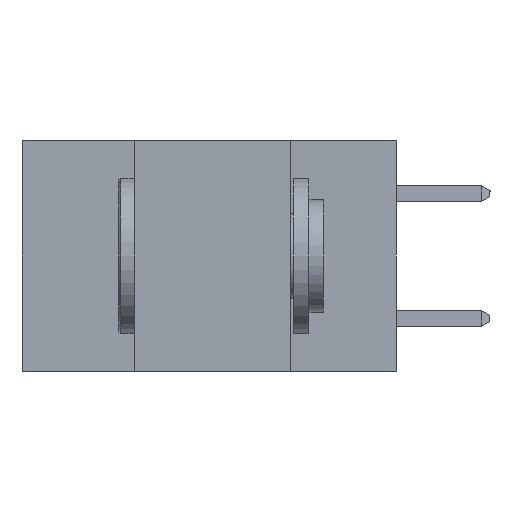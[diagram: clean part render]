
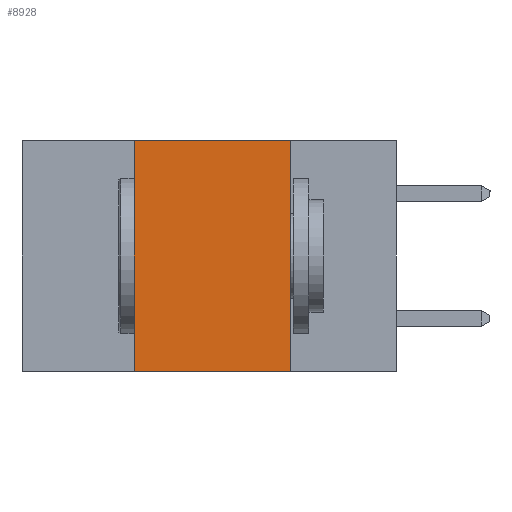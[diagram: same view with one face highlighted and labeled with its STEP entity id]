
A CAD part, left-side view. The second image highlights one B-rep face of the part: STEP entity #8928.
In plain terms, the highlighted planar face has unit normal (-1, 0, 0).
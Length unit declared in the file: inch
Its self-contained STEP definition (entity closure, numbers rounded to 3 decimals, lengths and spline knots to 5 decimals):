
#382 = EDGE_LOOP ( 'NONE', ( #12655, #15181, #7076, #5260 ) ) ;
#441 = VERTEX_POINT ( 'NONE', #9304 ) ;
#1180 = LINE ( 'NONE', #4933, #10960 ) ;
#1474 = VECTOR ( 'NONE', #10376, 39.37008 ) ;
#1528 = CARTESIAN_POINT ( 'NONE',  ( 0., 0.6, 0. ) ) ;
#1882 = AXIS2_PLACEMENT_3D ( 'NONE', #14109, #8125, #6566 ) ;
#2061 = DIRECTION ( 'NONE',  ( 0., 0., -1. ) ) ;
#2540 = LINE ( 'NONE', #1528, #10389 ) ;
#2710 = EDGE_CURVE ( 'NONE', #3416, #14634, #12738, .T. ) ;
#3416 = VERTEX_POINT ( 'NONE', #5160 ) ;
#3447 = DIRECTION ( 'NONE',  ( 0., -1., 0. ) ) ;
#4645 = CARTESIAN_POINT ( 'NONE',  ( 0., 0.42, 0. ) ) ;
#4933 = CARTESIAN_POINT ( 'NONE',  ( 0., 0.6, -0.37 ) ) ;
#5160 = CARTESIAN_POINT ( 'NONE',  ( 0., 0.42, -0.37 ) ) ;
#5260 = ORIENTED_EDGE ( 'NONE', *, *, #10572, .T. ) ;
#5879 = VECTOR ( 'NONE', #2061, 39.37008 ) ;
#6272 = EDGE_CURVE ( 'NONE', #441, #8677, #11792, .T. ) ;
#6566 = DIRECTION ( 'NONE',  ( 0., 0., -1. ) ) ;
#6716 = PLANE ( 'NONE',  #1882 ) ;
#7076 = ORIENTED_EDGE ( 'NONE', *, *, #2710, .F. ) ;
#7812 = EDGE_CURVE ( 'NONE', #14634, #441, #2540, .T. ) ;
#8125 = DIRECTION ( 'NONE',  ( 1., 0., 0. ) ) ;
#8677 = VERTEX_POINT ( 'NONE', #13109 ) ;
#8928 = ADVANCED_FACE ( 'NONE', ( #11424 ), #6716, .F. ) ;
#9304 = CARTESIAN_POINT ( 'NONE',  ( 0., 0.17, 0. ) ) ;
#10376 = DIRECTION ( 'NONE',  ( 0., 0., 1. ) ) ;
#10389 = VECTOR ( 'NONE', #12110, 39.37008 ) ;
#10572 = EDGE_CURVE ( 'NONE', #3416, #8677, #1180, .T. ) ;
#10960 = VECTOR ( 'NONE', #3447, 39.37008 ) ;
#11314 = CARTESIAN_POINT ( 'NONE',  ( 0., 0.42, -0.37 ) ) ;
#11424 = FACE_OUTER_BOUND ( 'NONE', #382, .T. ) ;
#11792 = LINE ( 'NONE', #12819, #5879 ) ;
#12110 = DIRECTION ( 'NONE',  ( 0., -1., 0. ) ) ;
#12655 = ORIENTED_EDGE ( 'NONE', *, *, #6272, .F. ) ;
#12738 = LINE ( 'NONE', #11314, #1474 ) ;
#12819 = CARTESIAN_POINT ( 'NONE',  ( 0., 0.17, -0.37 ) ) ;
#13109 = CARTESIAN_POINT ( 'NONE',  ( 0., 0.17, -0.37 ) ) ;
#14109 = CARTESIAN_POINT ( 'NONE',  ( 0., 0.6, 0. ) ) ;
#14634 = VERTEX_POINT ( 'NONE', #4645 ) ;
#15181 = ORIENTED_EDGE ( 'NONE', *, *, #7812, .F. ) ;
